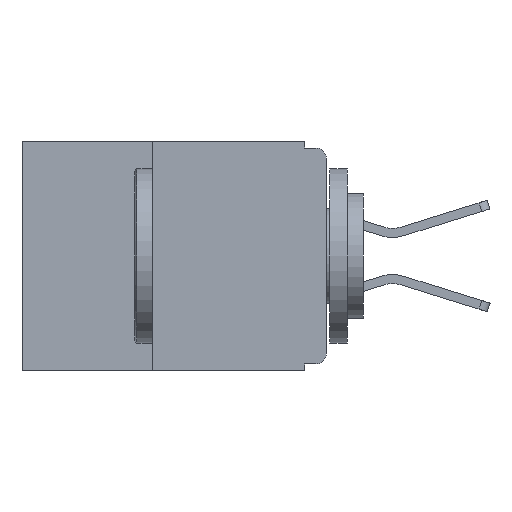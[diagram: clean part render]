
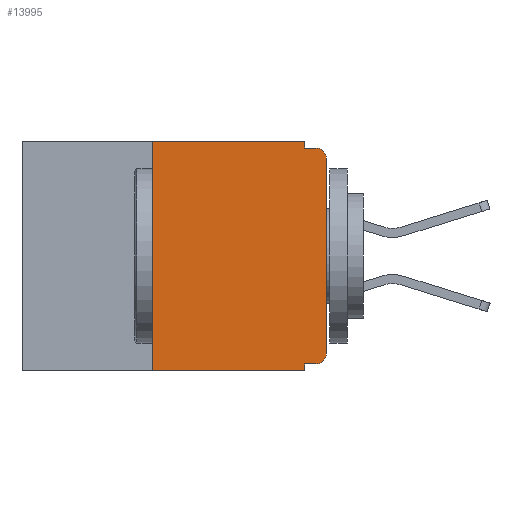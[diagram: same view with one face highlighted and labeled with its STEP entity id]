
A CAD part, left-side view. The second image highlights one B-rep face of the part: STEP entity #13995.
In plain terms, the highlighted planar face has unit normal (-1, 0, 0).
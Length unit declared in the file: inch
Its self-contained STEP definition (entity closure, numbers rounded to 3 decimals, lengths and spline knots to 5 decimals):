
#158 = ORIENTED_EDGE ( 'NONE', *, *, #27279, .T. ) ;
#395 = DIRECTION ( 'NONE',  ( 1., 0., 0. ) ) ;
#498 = DIRECTION ( 'NONE',  ( 0., 0., -1. ) ) ;
#680 = ORIENTED_EDGE ( 'NONE', *, *, #5677, .F. ) ;
#753 = ORIENTED_EDGE ( 'NONE', *, *, #17486, .F. ) ;
#915 = LINE ( 'NONE', #13719, #30534 ) ;
#1351 = DIRECTION ( 'NONE',  ( 0., 0., -1. ) ) ;
#1922 = LINE ( 'NONE', #6330, #29806 ) ;
#2138 = VERTEX_POINT ( 'NONE', #34687 ) ;
#2474 = DIRECTION ( 'NONE',  ( 0., 1., 0. ) ) ;
#3071 = DIRECTION ( 'NONE',  ( -1., 0., 0. ) ) ;
#3581 = ORIENTED_EDGE ( 'NONE', *, *, #27108, .F. ) ;
#4483 = VERTEX_POINT ( 'NONE', #9457 ) ;
#4544 = EDGE_CURVE ( 'NONE', #32385, #34667, #1922, .T. ) ;
#5034 = EDGE_LOOP ( 'NONE', ( #9751, #158, #680, #753, #3581, #10768, #14432, #17331, #21027, #22983 ) ) ;
#5677 = EDGE_CURVE ( 'NONE', #29557, #19091, #30977, .T. ) ;
#5931 = EDGE_CURVE ( 'NONE', #15125, #2138, #915, .T. ) ;
#6330 = CARTESIAN_POINT ( 'NONE',  ( 0., 0., 0. ) ) ;
#6747 = VECTOR ( 'NONE', #16608, 39.37008 ) ;
#7127 = EDGE_CURVE ( 'NONE', #10608, #12311, #18525, .T. ) ;
#7654 = AXIS2_PLACEMENT_3D ( 'NONE', #19998, #3071, #22717 ) ;
#7995 = VECTOR ( 'NONE', #18460, 39.37008 ) ;
#8000 = LINE ( 'NONE', #31155, #30121 ) ;
#8540 = VECTOR ( 'NONE', #498, 39.37008 ) ;
#8598 = DIRECTION ( 'NONE',  ( 0., 0., 1. ) ) ;
#9271 = EDGE_CURVE ( 'NONE', #12311, #4483, #23429, .T. ) ;
#9457 = CARTESIAN_POINT ( 'NONE',  ( 0., 0.031, -0.33 ) ) ;
#9751 = ORIENTED_EDGE ( 'NONE', *, *, #4544, .T. ) ;
#9781 = EDGE_CURVE ( 'NONE', #15125, #4483, #28912, .T. ) ;
#10608 = VERTEX_POINT ( 'NONE', #17185 ) ;
#10768 = ORIENTED_EDGE ( 'NONE', *, *, #5931, .F. ) ;
#12311 = VERTEX_POINT ( 'NONE', #27508 ) ;
#13029 = AXIS2_PLACEMENT_3D ( 'NONE', #14476, #395, #20139 ) ;
#13325 = LINE ( 'NONE', #32794, #27183 ) ;
#13719 = CARTESIAN_POINT ( 'NONE',  ( 0., 0.25, -0.33 ) ) ;
#13769 = CARTESIAN_POINT ( 'NONE',  ( 0., 0.25, -0.33 ) ) ;
#13829 = DIRECTION ( 'NONE',  ( 0., 0., 1. ) ) ;
#13974 = FACE_OUTER_BOUND ( 'NONE', #5034, .T. ) ;
#13995 = ADVANCED_FACE ( 'NONE', ( #13974 ), #30933, .F. ) ;
#14432 = ORIENTED_EDGE ( 'NONE', *, *, #9781, .T. ) ;
#14476 = CARTESIAN_POINT ( 'NONE',  ( 0., 0.437, 0. ) ) ;
#14709 = DIRECTION ( 'NONE',  ( 0., -1., 0. ) ) ;
#15125 = VERTEX_POINT ( 'NONE', #13769 ) ;
#16509 = CARTESIAN_POINT ( 'NONE',  ( 0., 0., -0.025 ) ) ;
#16608 = DIRECTION ( 'NONE',  ( 0., -1., 0. ) ) ;
#16938 = AXIS2_PLACEMENT_3D ( 'NONE', #34579, #18305, #1351 ) ;
#17185 = CARTESIAN_POINT ( 'NONE',  ( 0., 0.015, -0.32 ) ) ;
#17331 = ORIENTED_EDGE ( 'NONE', *, *, #9271, .F. ) ;
#17486 = EDGE_CURVE ( 'NONE', #33905, #29557, #13325, .T. ) ;
#18305 = DIRECTION ( 'NONE',  ( -1., 0., 0. ) ) ;
#18460 = DIRECTION ( 'NONE',  ( 0., -1., 0. ) ) ;
#18525 = LINE ( 'NONE', #19418, #32140 ) ;
#18565 = CARTESIAN_POINT ( 'NONE',  ( 0., 0., -0.01 ) ) ;
#19091 = VERTEX_POINT ( 'NONE', #24845 ) ;
#19418 = CARTESIAN_POINT ( 'NONE',  ( 0., 0., -0.32 ) ) ;
#19949 = CARTESIAN_POINT ( 'NONE',  ( 0., 0.031, -0.01 ) ) ;
#19998 = CARTESIAN_POINT ( 'NONE',  ( 0., 0.015, -0.305 ) ) ;
#20139 = DIRECTION ( 'NONE',  ( 0., 0., -1. ) ) ;
#21027 = ORIENTED_EDGE ( 'NONE', *, *, #7127, .F. ) ;
#22717 = DIRECTION ( 'NONE',  ( 0., 0., -1. ) ) ;
#22983 = ORIENTED_EDGE ( 'NONE', *, *, #35752, .T. ) ;
#23429 = LINE ( 'NONE', #33744, #8540 ) ;
#24803 = CARTESIAN_POINT ( 'NONE',  ( 0., 0.437, -0.33 ) ) ;
#24845 = CARTESIAN_POINT ( 'NONE',  ( 0., 0.015, -0.01 ) ) ;
#27108 = EDGE_CURVE ( 'NONE', #2138, #33905, #8000, .T. ) ;
#27183 = VECTOR ( 'NONE', #30039, 39.37008 ) ;
#27279 = EDGE_CURVE ( 'NONE', #34667, #19091, #32246, .T. ) ;
#27508 = CARTESIAN_POINT ( 'NONE',  ( 0., 0.031, -0.32 ) ) ;
#27660 = CARTESIAN_POINT ( 'NONE',  ( 0., 0., -0.305 ) ) ;
#28912 = LINE ( 'NONE', #24803, #6747 ) ;
#29557 = VERTEX_POINT ( 'NONE', #19949 ) ;
#29806 = VECTOR ( 'NONE', #8598, 39.37008 ) ;
#30039 = DIRECTION ( 'NONE',  ( 0., 0., -1. ) ) ;
#30121 = VECTOR ( 'NONE', #14709, 39.37008 ) ;
#30534 = VECTOR ( 'NONE', #13829, 39.37008 ) ;
#30933 = PLANE ( 'NONE',  #13029 ) ;
#30977 = LINE ( 'NONE', #18565, #7995 ) ;
#31155 = CARTESIAN_POINT ( 'NONE',  ( 0., 0.437, 0. ) ) ;
#32140 = VECTOR ( 'NONE', #2474, 39.37008 ) ;
#32246 = CIRCLE ( 'NONE', #16938, 0.015 ) ;
#32344 = CARTESIAN_POINT ( 'NONE',  ( 0., 0.031, 0. ) ) ;
#32385 = VERTEX_POINT ( 'NONE', #27660 ) ;
#32794 = CARTESIAN_POINT ( 'NONE',  ( 0., 0.031, 0. ) ) ;
#33744 = CARTESIAN_POINT ( 'NONE',  ( 0., 0.031, -0.33 ) ) ;
#33905 = VERTEX_POINT ( 'NONE', #32344 ) ;
#34579 = CARTESIAN_POINT ( 'NONE',  ( 0., 0.015, -0.025 ) ) ;
#34667 = VERTEX_POINT ( 'NONE', #16509 ) ;
#34686 = CIRCLE ( 'NONE', #7654, 0.015 ) ;
#34687 = CARTESIAN_POINT ( 'NONE',  ( 0., 0.25, 0. ) ) ;
#35752 = EDGE_CURVE ( 'NONE', #10608, #32385, #34686, .T. ) ;
